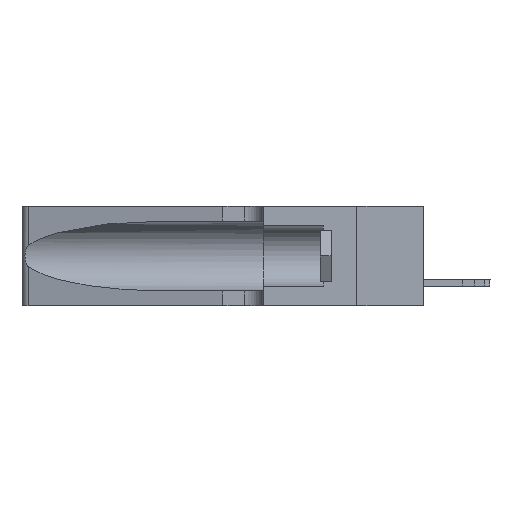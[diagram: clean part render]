
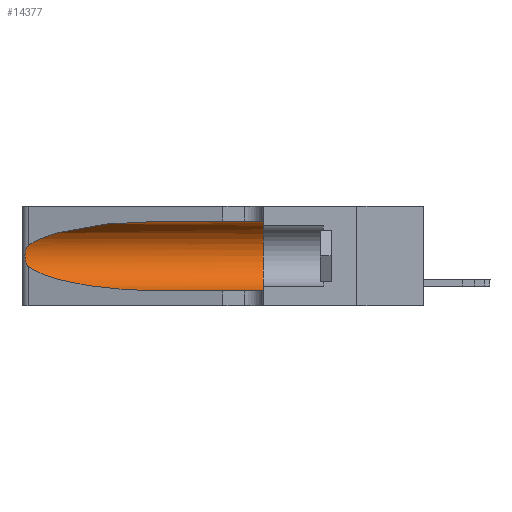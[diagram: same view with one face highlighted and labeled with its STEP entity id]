
A CAD part, left-side view. The second image highlights one B-rep face of the part: STEP entity #14377.
In plain terms, the highlighted cylindrical face has radius 3.308 mm (diameter 6.617 mm), a partial arc.
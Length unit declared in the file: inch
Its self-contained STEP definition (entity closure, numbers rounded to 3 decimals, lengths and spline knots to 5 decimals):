
#108 = FACE_OUTER_BOUND ( 'NONE', #9457, .T. ) ;
#389 = B_SPLINE_CURVE_WITH_KNOTS ( 'NONE', 3,
 ( #15095, #17913, #10890, #3875, #14967, #6507, #16610, #5323, #897, #16424, #5200, #2578, #3817, #6751 ),
 .UNSPECIFIED., .F., .F.,
 ( 4, 2, 2, 2, 2, 2, 4 ),
 ( 0., 0.00027, 0.00053, 0.00107, 0.0016, 0.00187, 0.00214 ),
 .UNSPECIFIED. ) ;
#897 = CARTESIAN_POINT ( 'NONE',  ( 0.26017, 1.23833, 0.17102 ) ) ;
#1028 = ORIENTED_EDGE ( 'NONE', *, *, #15380, .F. ) ;
#1270 = VERTEX_POINT ( 'NONE', #17376 ) ;
#1468 = ORIENTED_EDGE ( 'NONE', *, *, #3290, .T. ) ;
#2057 = VECTOR ( 'NONE', #13240, 39.37008 ) ;
#2105 = CARTESIAN_POINT ( 'NONE',  ( 0.25487, 1.22718, 0.22369 ) ) ;
#2301 =( BOUNDED_CURVE ( )  B_SPLINE_CURVE ( 3, ( #16623, #8204, #8323, #18175 ),
 .UNSPECIFIED., .F., .F. ) 
 B_SPLINE_CURVE_WITH_KNOTS ( ( 4, 4 ),
 ( 1.5708, 2.84003 ),
 .UNSPECIFIED. ) 
 CURVE ( )  GEOMETRIC_REPRESENTATION_ITEM ( )  RATIONAL_B_SPLINE_CURVE ( ( 1., 0.87, 0.87, 1. ) ) 
 REPRESENTATION_ITEM ( '' )  );
#2346 = CARTESIAN_POINT ( 'NONE',  ( 0.1305, 0.35, 0.185 ) ) ;
#2578 = CARTESIAN_POINT ( 'NONE',  ( 0.25639, 1.23186, 0.15144 ) ) ;
#3011 = VERTEX_POINT ( 'NONE', #3172 ) ;
#3172 = CARTESIAN_POINT ( 'NONE',  ( 0.1305, 0.35, 0.31525 ) ) ;
#3201 = DIRECTION ( 'NONE',  ( 0., -1., 0. ) ) ;
#3290 = EDGE_CURVE ( 'NONE', #8775, #1270, #13286, .T. ) ;
#3817 = CARTESIAN_POINT ( 'NONE',  ( 0.25555, 1.22993, 0.14849 ) ) ;
#3875 = CARTESIAN_POINT ( 'NONE',  ( 0.25787, 1.23484, 0.2124 ) ) ;
#4115 = AXIS2_PLACEMENT_3D ( 'NONE', #2346, #6594, #16443 ) ;
#5200 = CARTESIAN_POINT ( 'NONE',  ( 0.25789, 1.23486, 0.15765 ) ) ;
#5323 = CARTESIAN_POINT ( 'NONE',  ( 0.26075, 1.23896, 0.178 ) ) ;
#5548 = AXIS2_PLACEMENT_3D ( 'NONE', #17852, #12207, #15032 ) ;
#6232 = LINE ( 'NONE', #8985, #2057 ) ;
#6507 = CARTESIAN_POINT ( 'NONE',  ( 0.26018, 1.23835, 0.19895 ) ) ;
#6594 = DIRECTION ( 'NONE',  ( 0., 1., 0. ) ) ;
#6751 = CARTESIAN_POINT ( 'NONE',  ( 0.25487, 1.22718, 0.14631 ) ) ;
#6816 = CARTESIAN_POINT ( 'NONE',  ( 0.1305, 0.72297, 0.05475 ) ) ;
#6858 = EDGE_CURVE ( 'NONE', #17902, #11738, #2301, .T. ) ;
#7935 = VERTEX_POINT ( 'NONE', #12529 ) ;
#7961 = EDGE_CURVE ( 'NONE', #1270, #7935, #11544, .T. ) ;
#8204 = CARTESIAN_POINT ( 'NONE',  ( 0.18966, 0.96281, 0.31525 ) ) ;
#8323 = CARTESIAN_POINT ( 'NONE',  ( 0.2373, 1.15595, 0.28018 ) ) ;
#8775 = VERTEX_POINT ( 'NONE', #15188 ) ;
#8985 = CARTESIAN_POINT ( 'NONE',  ( 0.1305, 1.61858, 0.31525 ) ) ;
#9457 = EDGE_LOOP ( 'NONE', ( #12950, #14120, #1468, #11054, #14764, #1028 ) ) ;
#10890 = CARTESIAN_POINT ( 'NONE',  ( 0.25639, 1.23184, 0.21858 ) ) ;
#10954 = CARTESIAN_POINT ( 'NONE',  ( 0.2373, 1.15595, 0.08982 ) ) ;
#11054 = ORIENTED_EDGE ( 'NONE', *, *, #7961, .T. ) ;
#11544 = LINE ( 'NONE', #15754, #16147 ) ;
#11738 = VERTEX_POINT ( 'NONE', #2105 ) ;
#12207 = DIRECTION ( 'NONE',  ( 0., -1., 0. ) ) ;
#12394 = CARTESIAN_POINT ( 'NONE',  ( 0.18966, 0.96281, 0.05475 ) ) ;
#12529 = CARTESIAN_POINT ( 'NONE',  ( 0.1305, 0.35, 0.05475 ) ) ;
#12950 = ORIENTED_EDGE ( 'NONE', *, *, #6858, .T. ) ;
#13240 = DIRECTION ( 'NONE',  ( 0., -1., 0. ) ) ;
#13286 =( BOUNDED_CURVE ( )  B_SPLINE_CURVE ( 3, ( #14571, #10954, #12394, #6816 ),
 .UNSPECIFIED., .F., .T. ) 
 B_SPLINE_CURVE_WITH_KNOTS ( ( 4, 4 ),
 ( 3.44316, 4.71239 ),
 .UNSPECIFIED. ) 
 CURVE ( )  GEOMETRIC_REPRESENTATION_ITEM ( )  RATIONAL_B_SPLINE_CURVE ( ( 1., 0.87, 0.87, 1. ) ) 
 REPRESENTATION_ITEM ( '' )  );
#14120 = ORIENTED_EDGE ( 'NONE', *, *, #16889, .T. ) ;
#14377 = ADVANCED_FACE ( 'NONE', ( #108 ), #16876, .F. ) ;
#14455 = CARTESIAN_POINT ( 'NONE',  ( 0.1305, 0.72297, 0.31525 ) ) ;
#14571 = CARTESIAN_POINT ( 'NONE',  ( 0.25487, 1.22718, 0.14631 ) ) ;
#14764 = ORIENTED_EDGE ( 'NONE', *, *, #16278, .F. ) ;
#14967 = CARTESIAN_POINT ( 'NONE',  ( 0.25854, 1.2359, 0.20912 ) ) ;
#15032 = DIRECTION ( 'NONE',  ( 0., 0., -1. ) ) ;
#15095 = CARTESIAN_POINT ( 'NONE',  ( 0.25487, 1.22718, 0.22369 ) ) ;
#15188 = CARTESIAN_POINT ( 'NONE',  ( 0.25487, 1.22718, 0.14631 ) ) ;
#15380 = EDGE_CURVE ( 'NONE', #17902, #3011, #6232, .T. ) ;
#15754 = CARTESIAN_POINT ( 'NONE',  ( 0.1305, 1.61858, 0.05475 ) ) ;
#16147 = VECTOR ( 'NONE', #3201, 39.37008 ) ;
#16278 = EDGE_CURVE ( 'NONE', #3011, #7935, #17654, .T. ) ;
#16424 = CARTESIAN_POINT ( 'NONE',  ( 0.25856, 1.23593, 0.16098 ) ) ;
#16443 = DIRECTION ( 'NONE',  ( 0., 0., 1. ) ) ;
#16610 = CARTESIAN_POINT ( 'NONE',  ( 0.26075, 1.23896, 0.19203 ) ) ;
#16623 = CARTESIAN_POINT ( 'NONE',  ( 0.1305, 0.72297, 0.31525 ) ) ;
#16876 = CYLINDRICAL_SURFACE ( 'NONE', #5548, 0.13025 ) ;
#16889 = EDGE_CURVE ( 'NONE', #11738, #8775, #389, .T. ) ;
#17376 = CARTESIAN_POINT ( 'NONE',  ( 0.1305, 0.72297, 0.05475 ) ) ;
#17654 = CIRCLE ( 'NONE', #4115, 0.13025 ) ;
#17852 = CARTESIAN_POINT ( 'NONE',  ( 0.1305, 1.61858, 0.185 ) ) ;
#17902 = VERTEX_POINT ( 'NONE', #14455 ) ;
#17913 = CARTESIAN_POINT ( 'NONE',  ( 0.25555, 1.22994, 0.2215 ) ) ;
#18175 = CARTESIAN_POINT ( 'NONE',  ( 0.25487, 1.22718, 0.22369 ) ) ;
